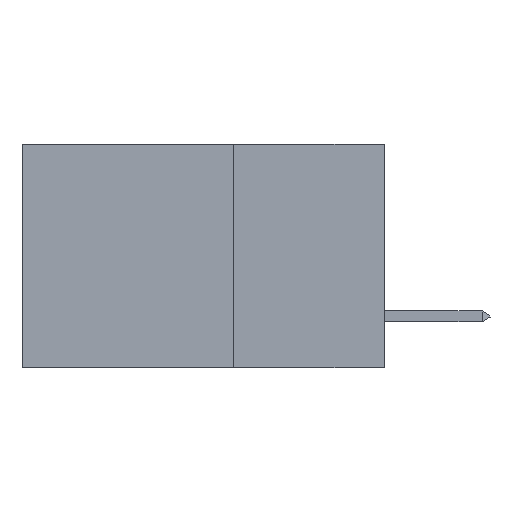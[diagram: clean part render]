
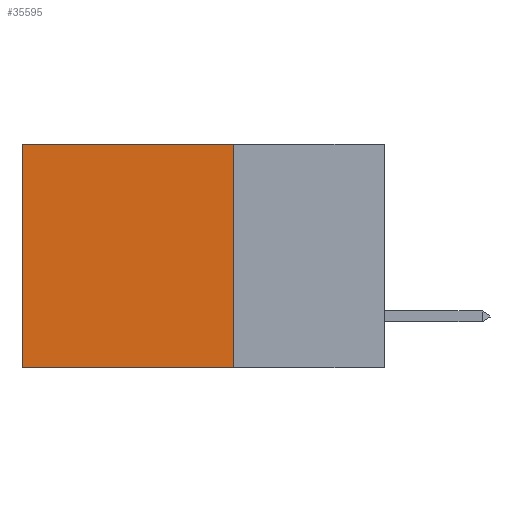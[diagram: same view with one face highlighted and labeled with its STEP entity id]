
A CAD part, left-side view. The second image highlights one B-rep face of the part: STEP entity #35595.
In plain terms, the highlighted planar face has unit normal (-1, 0, 0).
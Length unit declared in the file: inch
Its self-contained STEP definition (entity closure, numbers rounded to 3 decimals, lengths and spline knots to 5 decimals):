
#1149 = EDGE_LOOP ( 'NONE', ( #2565, #19041, #29452, #1522 ) ) ;
#1522 = ORIENTED_EDGE ( 'NONE', *, *, #23555, .T. ) ;
#2565 = ORIENTED_EDGE ( 'NONE', *, *, #39061, .T. ) ;
#5407 = VECTOR ( 'NONE', #34061, 39.37008 ) ;
#6555 = CARTESIAN_POINT ( 'NONE',  ( 0.2875, 0.6, 0. ) ) ;
#7098 = VERTEX_POINT ( 'NONE', #6555 ) ;
#9978 = CARTESIAN_POINT ( 'NONE',  ( 0.2875, 0.6, -0.37 ) ) ;
#10690 = VECTOR ( 'NONE', #29503, 39.37008 ) ;
#11361 = LINE ( 'NONE', #22771, #38269 ) ;
#11766 = LINE ( 'NONE', #25754, #21659 ) ;
#14301 = DIRECTION ( 'NONE',  ( 0., 0., -1. ) ) ;
#16256 = CARTESIAN_POINT ( 'NONE',  ( 0.2875, 0.25, -0.37 ) ) ;
#17226 = CARTESIAN_POINT ( 'NONE',  ( 0.2875, 0.25, 0. ) ) ;
#17770 = LINE ( 'NONE', #32126, #10690 ) ;
#17894 = AXIS2_PLACEMENT_3D ( 'NONE', #17226, #22992, #14301 ) ;
#18625 = LINE ( 'NONE', #33822, #5407 ) ;
#19041 = ORIENTED_EDGE ( 'NONE', *, *, #30965, .F. ) ;
#19356 = CARTESIAN_POINT ( 'NONE',  ( 0.2875, 0.25, 0. ) ) ;
#21659 = VECTOR ( 'NONE', #31836, 39.37008 ) ;
#22771 = CARTESIAN_POINT ( 'NONE',  ( 0.2875, 0.25, 0. ) ) ;
#22992 = DIRECTION ( 'NONE',  ( 1., 0., 0. ) ) ;
#23003 = VERTEX_POINT ( 'NONE', #19356 ) ;
#23555 = EDGE_CURVE ( 'NONE', #23003, #7098, #18625, .T. ) ;
#25754 = CARTESIAN_POINT ( 'NONE',  ( 0.2875, 0.25, -0.37 ) ) ;
#25808 = DIRECTION ( 'NONE',  ( 0., 0., -1. ) ) ;
#26721 = VERTEX_POINT ( 'NONE', #16256 ) ;
#29452 = ORIENTED_EDGE ( 'NONE', *, *, #35996, .F. ) ;
#29503 = DIRECTION ( 'NONE',  ( 0., 0., -1. ) ) ;
#30744 = FACE_OUTER_BOUND ( 'NONE', #1149, .T. ) ;
#30965 = EDGE_CURVE ( 'NONE', #26721, #38758, #11766, .T. ) ;
#31836 = DIRECTION ( 'NONE',  ( 0., 1., 0. ) ) ;
#32126 = CARTESIAN_POINT ( 'NONE',  ( 0.2875, 0.6, 0. ) ) ;
#33822 = CARTESIAN_POINT ( 'NONE',  ( 0.2875, 0.25, 0. ) ) ;
#34061 = DIRECTION ( 'NONE',  ( 0., 1., 0. ) ) ;
#35595 = ADVANCED_FACE ( 'NONE', ( #30744 ), #38564, .F. ) ;
#35996 = EDGE_CURVE ( 'NONE', #23003, #26721, #11361, .T. ) ;
#38269 = VECTOR ( 'NONE', #25808, 39.37008 ) ;
#38564 = PLANE ( 'NONE',  #17894 ) ;
#38758 = VERTEX_POINT ( 'NONE', #9978 ) ;
#39061 = EDGE_CURVE ( 'NONE', #7098, #38758, #17770, .T. ) ;
